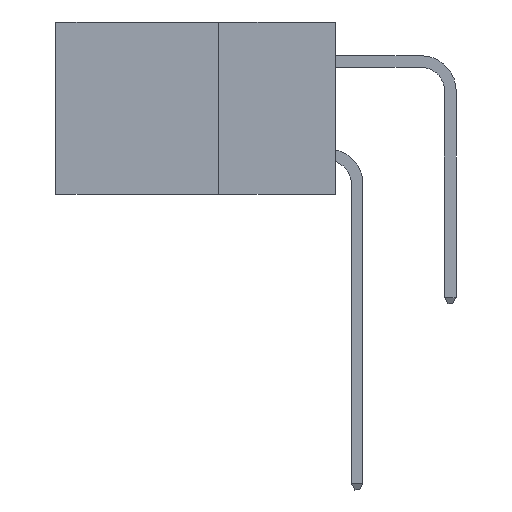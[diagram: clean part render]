
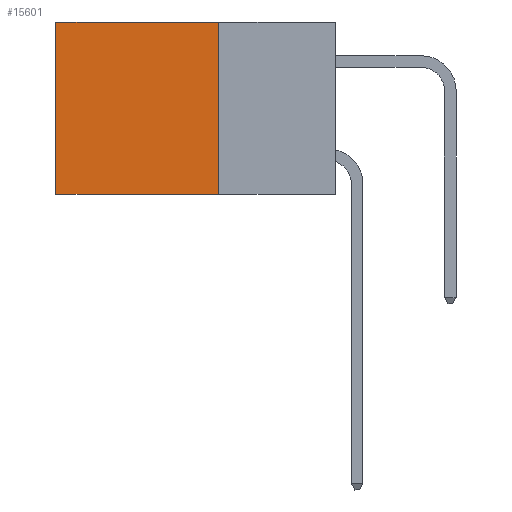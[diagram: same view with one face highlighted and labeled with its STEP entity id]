
A CAD part, left-side view. The second image highlights one B-rep face of the part: STEP entity #15601.
In plain terms, the highlighted planar face has unit normal (-1, 0, 0).
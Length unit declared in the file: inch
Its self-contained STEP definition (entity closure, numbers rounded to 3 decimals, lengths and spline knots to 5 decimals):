
#1175 = VECTOR ( 'NONE', #15880, 39.37008 ) ;
#2366 = EDGE_CURVE ( 'NONE', #4684, #3594, #5338, .T. ) ;
#2877 = PLANE ( 'NONE',  #11613 ) ;
#3211 = EDGE_CURVE ( 'NONE', #30285, #29667, #7509, .T. ) ;
#3594 = VERTEX_POINT ( 'NONE', #24847 ) ;
#4684 = VERTEX_POINT ( 'NONE', #21678 ) ;
#5279 = CARTESIAN_POINT ( 'NONE',  ( 0.2875, 0.25, 0. ) ) ;
#5338 = LINE ( 'NONE', #26456, #17178 ) ;
#7509 = LINE ( 'NONE', #13510, #1175 ) ;
#7650 = DIRECTION ( 'NONE',  ( 1., 0., 0. ) ) ;
#7835 = ORIENTED_EDGE ( 'NONE', *, *, #14597, .F. ) ;
#8181 = FACE_OUTER_BOUND ( 'NONE', #23224, .T. ) ;
#10104 = VECTOR ( 'NONE', #25400, 39.37008 ) ;
#11516 = LINE ( 'NONE', #24070, #16347 ) ;
#11613 = AXIS2_PLACEMENT_3D ( 'NONE', #5279, #7650, #24207 ) ;
#13510 = CARTESIAN_POINT ( 'NONE',  ( 0.2875, 0.25, 0. ) ) ;
#14489 = ORIENTED_EDGE ( 'NONE', *, *, #3211, .T. ) ;
#14597 = EDGE_CURVE ( 'NONE', #30285, #4684, #28957, .T. ) ;
#14610 = DIRECTION ( 'NONE',  ( 0., 1., 0. ) ) ;
#14908 = ORIENTED_EDGE ( 'NONE', *, *, #2366, .F. ) ;
#15601 = ADVANCED_FACE ( 'NONE', ( #8181 ), #2877, .F. ) ;
#15880 = DIRECTION ( 'NONE',  ( 0., 1., 0. ) ) ;
#16347 = VECTOR ( 'NONE', #26432, 39.37008 ) ;
#17178 = VECTOR ( 'NONE', #14610, 39.37008 ) ;
#18371 = CARTESIAN_POINT ( 'NONE',  ( 0.2875, 0.6, 0. ) ) ;
#20184 = ORIENTED_EDGE ( 'NONE', *, *, #20781, .T. ) ;
#20781 = EDGE_CURVE ( 'NONE', #29667, #3594, #11516, .T. ) ;
#21678 = CARTESIAN_POINT ( 'NONE',  ( 0.2875, 0.25, -0.37 ) ) ;
#23040 = CARTESIAN_POINT ( 'NONE',  ( 0.2875, 0.25, 0. ) ) ;
#23224 = EDGE_LOOP ( 'NONE', ( #20184, #14908, #7835, #14489 ) ) ;
#24070 = CARTESIAN_POINT ( 'NONE',  ( 0.2875, 0.6, 0. ) ) ;
#24207 = DIRECTION ( 'NONE',  ( 0., 0., -1. ) ) ;
#24847 = CARTESIAN_POINT ( 'NONE',  ( 0.2875, 0.6, -0.37 ) ) ;
#25400 = DIRECTION ( 'NONE',  ( 0., 0., -1. ) ) ;
#26432 = DIRECTION ( 'NONE',  ( 0., 0., -1. ) ) ;
#26456 = CARTESIAN_POINT ( 'NONE',  ( 0.2875, 0.25, -0.37 ) ) ;
#28957 = LINE ( 'NONE', #23040, #10104 ) ;
#29086 = CARTESIAN_POINT ( 'NONE',  ( 0.2875, 0.25, 0. ) ) ;
#29667 = VERTEX_POINT ( 'NONE', #18371 ) ;
#30285 = VERTEX_POINT ( 'NONE', #29086 ) ;
